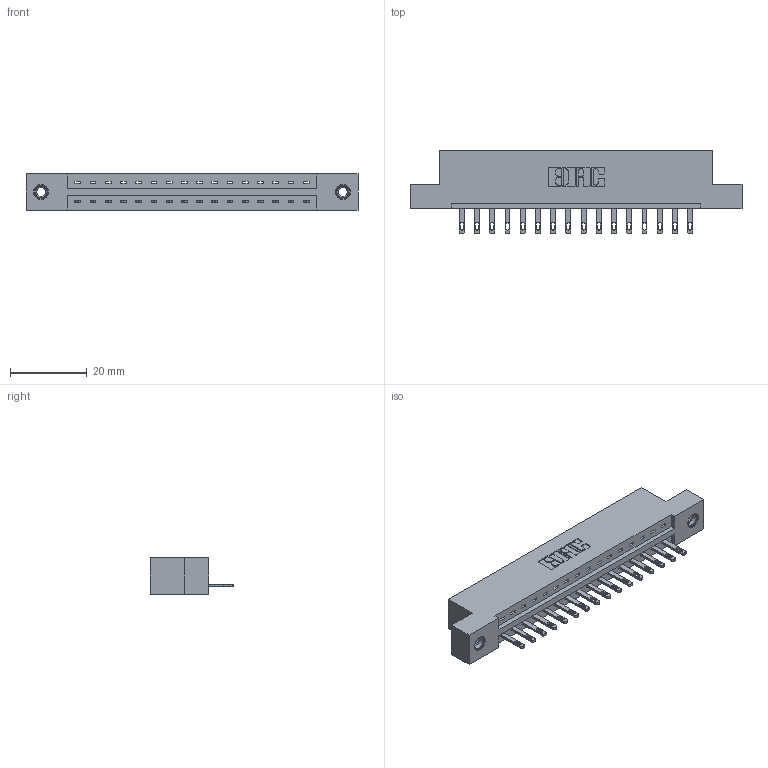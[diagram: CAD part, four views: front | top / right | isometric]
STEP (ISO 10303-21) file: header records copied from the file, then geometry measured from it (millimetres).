
FILE_DESCRIPTION (( 'STEP AP203' ), '1' );
FILE_NAME ('887-016-500-108.STEP', '2020-09-20T17:10:41', ( '' ), ( '' ), 'SwSTEP 2.0', 'SolidWorks 2020', '' );
FILE_SCHEMA (( 'CONFIG_CONTROL_DESIGN' ));
Length unit declared in the file: inch
Products named in the file (4): 345-292-001_345-293-100; 837 Part_Flush Mounting Lugs - 0.156 Dia-TI; 887-016-500-108; 345-250-001_345-250-003-102
Assembly tree (19 placements, depth 2):
  887-016-500-108
    837 Part_Flush Mounting Lugs - 0.156 Dia-TI
    345-292-001_345-293-100  x16
    345-250-001_345-250-003-102  x2
Bounding box: 86.41 x 21.85 x 9.4 mm (x, y, z)
Volume: 8659 mm3; surface area: 8870.5 mm2
Topology: 19 solids, 19 shells, 1102 faces, 3327 edges, 2210 vertices
Faces by surface type: plane 742, cylinder 344, cone 12, torus 4
Entity records: 16372 total; most frequent: CARTESIAN_POINT 2829, ORIENTED_EDGE 2774, DIRECTION 2469, EDGE_CURVE 1387, LINE 1235, VECTOR 1235, VERTEX_POINT 920, AXIS2_PLACEMENT_3D 617
